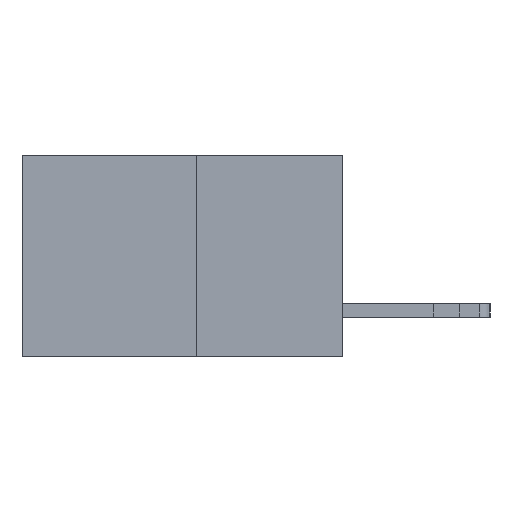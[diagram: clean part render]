
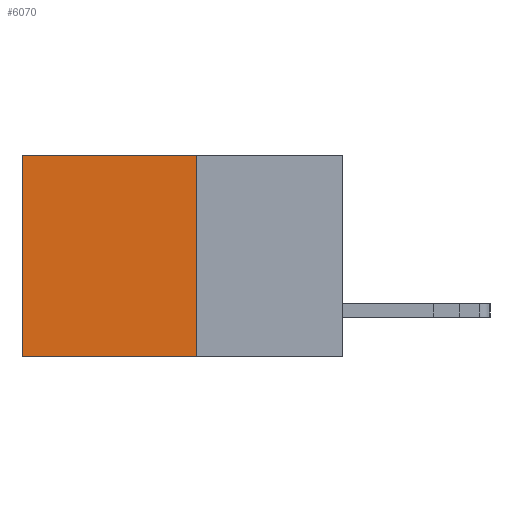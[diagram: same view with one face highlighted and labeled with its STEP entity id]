
A CAD part, left-side view. The second image highlights one B-rep face of the part: STEP entity #6070.
In plain terms, the highlighted planar face has unit normal (-1, 0, 0).
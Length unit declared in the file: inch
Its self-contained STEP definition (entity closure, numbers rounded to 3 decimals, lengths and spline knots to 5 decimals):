
#82 = AXIS2_PLACEMENT_3D ( 'NONE', #14321, #14118, #14091 ) ;
#127 = DIRECTION ( 'NONE',  ( 0., 1., 0. ) ) ;
#202 = CARTESIAN_POINT ( 'NONE',  ( 0.277, 0.27, 0. ) ) ;
#444 = DIRECTION ( 'NONE',  ( 0., 0., -1. ) ) ;
#561 = VERTEX_POINT ( 'NONE', #4443 ) ;
#750 = CARTESIAN_POINT ( 'NONE',  ( 0.277, 0.27, -0.37 ) ) ;
#1088 = EDGE_LOOP ( 'NONE', ( #10646, #14125, #4225, #7869 ) ) ;
#1548 = CARTESIAN_POINT ( 'NONE',  ( 0.277, 0.27, 0. ) ) ;
#2283 = VECTOR ( 'NONE', #9028, 39.37008 ) ;
#2970 = LINE ( 'NONE', #750, #8977 ) ;
#3724 = CARTESIAN_POINT ( 'NONE',  ( 0.277, 0.27, -0.37 ) ) ;
#3800 = EDGE_CURVE ( 'NONE', #561, #11681, #10908, .T. ) ;
#4225 = ORIENTED_EDGE ( 'NONE', *, *, #6015, .F. ) ;
#4443 = CARTESIAN_POINT ( 'NONE',  ( 0.277, 0.59, 0. ) ) ;
#5333 = VECTOR ( 'NONE', #127, 39.37008 ) ;
#5986 = VERTEX_POINT ( 'NONE', #1548 ) ;
#6010 = CARTESIAN_POINT ( 'NONE',  ( 0.277, 0.59, -0.37 ) ) ;
#6015 = EDGE_CURVE ( 'NONE', #5986, #12238, #2970, .T. ) ;
#6070 = ADVANCED_FACE ( 'NONE', ( #8289 ), #14154, .F. ) ;
#7606 = EDGE_CURVE ( 'NONE', #5986, #561, #11189, .T. ) ;
#7769 = LINE ( 'NONE', #3724, #10045 ) ;
#7869 = ORIENTED_EDGE ( 'NONE', *, *, #7606, .T. ) ;
#8289 = FACE_OUTER_BOUND ( 'NONE', #1088, .T. ) ;
#8977 = VECTOR ( 'NONE', #444, 39.37008 ) ;
#9028 = DIRECTION ( 'NONE',  ( 0., 0., -1. ) ) ;
#9070 = CARTESIAN_POINT ( 'NONE',  ( 0.277, 0.59, -0.37 ) ) ;
#10045 = VECTOR ( 'NONE', #11415, 39.37008 ) ;
#10646 = ORIENTED_EDGE ( 'NONE', *, *, #3800, .T. ) ;
#10908 = LINE ( 'NONE', #9070, #2283 ) ;
#11189 = LINE ( 'NONE', #202, #5333 ) ;
#11415 = DIRECTION ( 'NONE',  ( 0., 1., 0. ) ) ;
#11681 = VERTEX_POINT ( 'NONE', #6010 ) ;
#12238 = VERTEX_POINT ( 'NONE', #13551 ) ;
#12885 = EDGE_CURVE ( 'NONE', #12238, #11681, #7769, .T. ) ;
#13551 = CARTESIAN_POINT ( 'NONE',  ( 0.277, 0.27, -0.37 ) ) ;
#14091 = DIRECTION ( 'NONE',  ( 0., 0., -1. ) ) ;
#14118 = DIRECTION ( 'NONE',  ( 1., 0., 0. ) ) ;
#14125 = ORIENTED_EDGE ( 'NONE', *, *, #12885, .F. ) ;
#14154 = PLANE ( 'NONE',  #82 ) ;
#14321 = CARTESIAN_POINT ( 'NONE',  ( 0.277, 0.27, -0.37 ) ) ;
